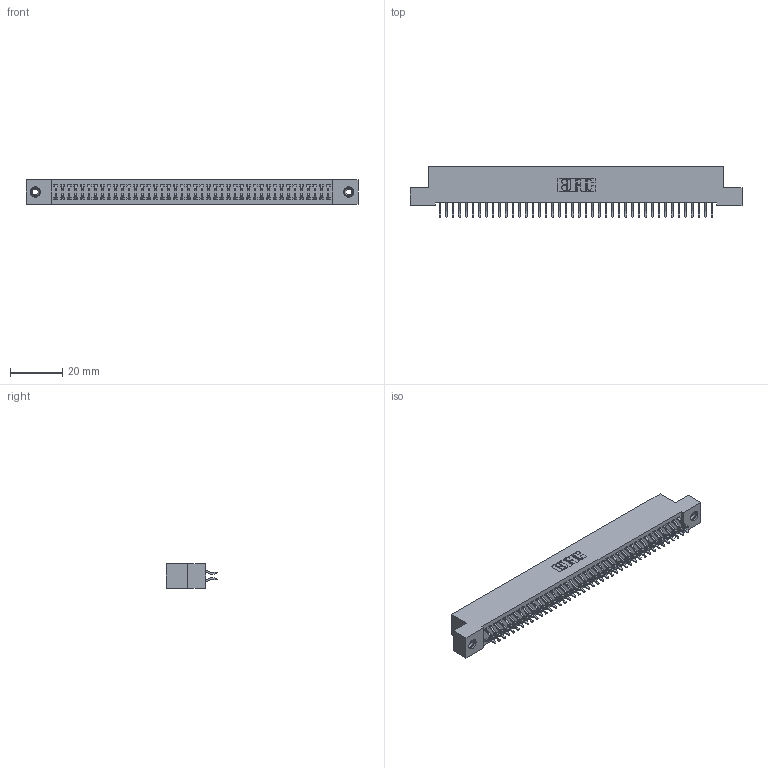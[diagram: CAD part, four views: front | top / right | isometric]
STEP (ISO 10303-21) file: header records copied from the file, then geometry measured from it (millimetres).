
FILE_DESCRIPTION (( 'STEP AP203' ), '1' );
FILE_NAME ('392-084-556-208.STEP', '2019-10-09T15:50:36', ( '' ), ( '' ), 'SwSTEP 2.0', 'SolidWorks 2016', '' );
FILE_SCHEMA (( 'CONFIG_CONTROL_DESIGN' ));
Length unit declared in the file: inch
Products named in the file (4): 342 Part_TI; 345-292-001_556 Tail; 345-250-001_345-250-003-102; 392-084-556-208
Assembly tree (87 placements, depth 2):
  392-084-556-208
    342 Part_TI
    345-292-001_556 Tail  x84
    345-250-001_345-250-003-102  x2
Bounding box: 127 x 19.58 x 9.4 mm (x, y, z)
Volume: 11403.1 mm3; surface area: 18490.2 mm2
Topology: 87 solids, 87 shells, 5042 faces, 14967 edges, 9858 vertices
Faces by surface type: plane 3458, cylinder 1568, cone 12, torus 4
Entity records: 28294 total; most frequent: CARTESIAN_POINT 4685, ORIENTED_EDGE 4602, DIRECTION 4023, EDGE_CURVE 2301, VECTOR 2145, LINE 2145, VERTEX_POINT 1528, AXIS2_PLACEMENT_3D 939
